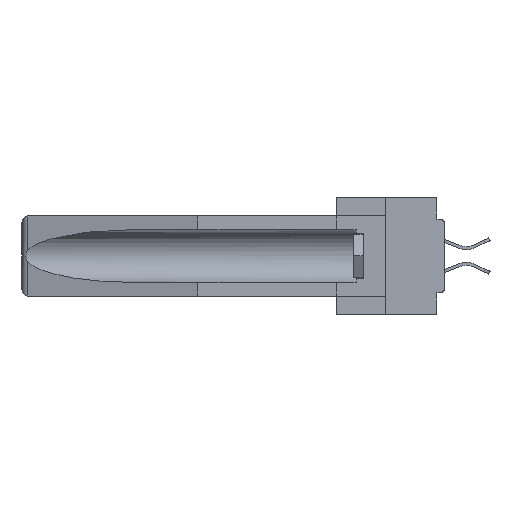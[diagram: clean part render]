
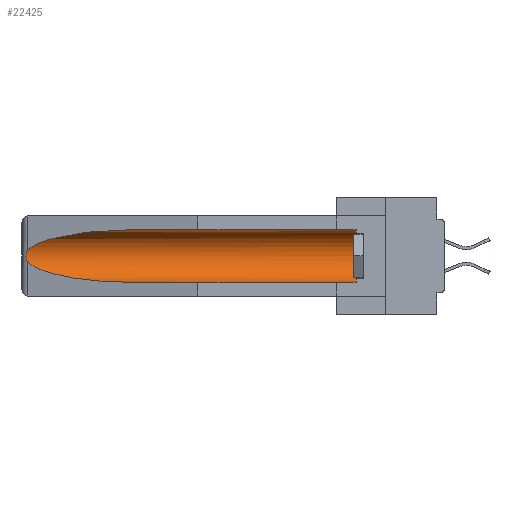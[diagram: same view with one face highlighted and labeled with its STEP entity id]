
A CAD part, left-side view. The second image highlights one B-rep face of the part: STEP entity #22425.
In plain terms, the highlighted cylindrical face has radius 2.857 mm (diameter 5.715 mm), a partial arc.
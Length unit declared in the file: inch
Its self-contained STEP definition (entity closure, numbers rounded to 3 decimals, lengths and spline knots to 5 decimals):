
#254 = CARTESIAN_POINT ( 'NONE',  ( 0.21114, 1.30732, -0.059 ) ) ;
#322 = EDGE_CURVE ( 'NONE', #24030, #15354, #25024, .T. ) ;
#728 = CARTESIAN_POINT ( 'NONE',  ( 0.2675, 1.53308, -0.16763 ) ) ;
#823 =( BOUNDED_CURVE ( )  B_SPLINE_CURVE ( 3, ( #20902, #254, #3367, #24155 ),
 .UNSPECIFIED., .F., .F. ) 
 B_SPLINE_CURVE_WITH_KNOTS ( ( 4, 4 ),
 ( 4.71239, 6.08839 ),
 .UNSPECIFIED. ) 
 CURVE ( )  GEOMETRIC_REPRESENTATION_ITEM ( )  RATIONAL_B_SPLINE_CURVE ( ( 1., 0.848, 0.848, 1. ) ) 
 REPRESENTATION_ITEM ( '' )  );
#825 = CYLINDRICAL_SURFACE ( 'NONE', #8034, 0.1125 ) ;
#1523 = B_SPLINE_CURVE_WITH_KNOTS ( 'NONE', 3,
 ( #2944, #11769, #5911, #36228, #728, #15561, #9840, #12424, #6300, #6419 ),
 .UNSPECIFIED., .F., .F.,
 ( 4, 2, 2, 2, 4 ),
 ( 0., 0.00029, 0.00058, 0.00087, 0.00117 ),
 .UNSPECIFIED. ) ;
#1564 = CARTESIAN_POINT ( 'NONE',  ( 0.155, -0.30754, -0.284 ) ) ;
#1683 = DIRECTION ( 'NONE',  ( 0., 1., 0. ) ) ;
#2037 = CARTESIAN_POINT ( 'NONE',  ( 0.155, 0.126, -0.1715 ) ) ;
#2944 = CARTESIAN_POINT ( 'NONE',  ( 0.26537, 1.52718, -0.14972 ) ) ;
#3367 = CARTESIAN_POINT ( 'NONE',  ( 0.25451, 1.48313, -0.09465 ) ) ;
#3453 = ORIENTED_EDGE ( 'NONE', *, *, #322, .T. ) ;
#4276 = VERTEX_POINT ( 'NONE', #21068 ) ;
#4538 = EDGE_LOOP ( 'NONE', ( #18793, #7656, #26432, #9390, #35405, #3453 ) ) ;
#5125 = CARTESIAN_POINT ( 'NONE',  ( 0.155, 1.07973, -0.284 ) ) ;
#5133 = DIRECTION ( 'NONE',  ( 0., 0., 1. ) ) ;
#5911 = CARTESIAN_POINT ( 'NONE',  ( 0.26654, 1.53092, -0.15636 ) ) ;
#6300 = CARTESIAN_POINT ( 'NONE',  ( 0.26597, 1.5296, -0.19026 ) ) ;
#6419 = CARTESIAN_POINT ( 'NONE',  ( 0.26537, 1.52718, -0.19328 ) ) ;
#6551 = DIRECTION ( 'NONE',  ( 0., 0., 1. ) ) ;
#6718 = CARTESIAN_POINT ( 'NONE',  ( 0.155, 1.07973, -0.059 ) ) ;
#7656 = ORIENTED_EDGE ( 'NONE', *, *, #36090, .T. ) ;
#8034 = AXIS2_PLACEMENT_3D ( 'NONE', #21124, #33382, #6551 ) ;
#9376 = CIRCLE ( 'NONE', #15101, 0.1125 ) ;
#9390 = ORIENTED_EDGE ( 'NONE', *, *, #18769, .F. ) ;
#9840 = CARTESIAN_POINT ( 'NONE',  ( 0.2673, 1.53269, -0.17917 ) ) ;
#11769 = CARTESIAN_POINT ( 'NONE',  ( 0.26597, 1.52961, -0.15275 ) ) ;
#12424 = CARTESIAN_POINT ( 'NONE',  ( 0.26655, 1.53094, -0.18657 ) ) ;
#12952 = CARTESIAN_POINT ( 'NONE',  ( 0.25451, 1.48313, -0.24835 ) ) ;
#13087 = CARTESIAN_POINT ( 'NONE',  ( 0.21114, 1.30732, -0.284 ) ) ;
#14111 = DIRECTION ( 'NONE',  ( 0., -1., 0. ) ) ;
#15101 = AXIS2_PLACEMENT_3D ( 'NONE', #2037, #14111, #5133 ) ;
#15354 = VERTEX_POINT ( 'NONE', #6718 ) ;
#15512 = CARTESIAN_POINT ( 'NONE',  ( 0.155, 0.126, -0.059 ) ) ;
#15561 = CARTESIAN_POINT ( 'NONE',  ( 0.2675, 1.53308, -0.17534 ) ) ;
#17628 = VECTOR ( 'NONE', #1683, 39.37008 ) ;
#18769 = EDGE_CURVE ( 'NONE', #21579, #19086, #25560, .T. ) ;
#18793 = ORIENTED_EDGE ( 'NONE', *, *, #18933, .T. ) ;
#18933 = EDGE_CURVE ( 'NONE', #15354, #36794, #823, .T. ) ;
#19086 = VERTEX_POINT ( 'NONE', #5125 ) ;
#20902 = CARTESIAN_POINT ( 'NONE',  ( 0.155, 1.07973, -0.059 ) ) ;
#21068 = CARTESIAN_POINT ( 'NONE',  ( 0.26537, 1.52718, -0.19328 ) ) ;
#21124 = CARTESIAN_POINT ( 'NONE',  ( 0.155, -0.30754, -0.1715 ) ) ;
#21579 = VERTEX_POINT ( 'NONE', #31750 ) ;
#21800 = CARTESIAN_POINT ( 'NONE',  ( 0.26537, 1.52718, -0.19328 ) ) ;
#22425 = ADVANCED_FACE ( 'NONE', ( #36643 ), #825, .F. ) ;
#23085 = VECTOR ( 'NONE', #34253, 39.37008 ) ;
#24030 = VERTEX_POINT ( 'NONE', #15512 ) ;
#24155 = CARTESIAN_POINT ( 'NONE',  ( 0.26537, 1.52718, -0.14972 ) ) ;
#25024 = LINE ( 'NONE', #33743, #23085 ) ;
#25560 = LINE ( 'NONE', #1564, #17628 ) ;
#25986 = EDGE_CURVE ( 'NONE', #4276, #19086, #29712, .T. ) ;
#26432 = ORIENTED_EDGE ( 'NONE', *, *, #25986, .T. ) ;
#29712 =( BOUNDED_CURVE ( )  B_SPLINE_CURVE ( 3, ( #21800, #12952, #13087, #36904 ),
 .UNSPECIFIED., .F., .F. ) 
 B_SPLINE_CURVE_WITH_KNOTS ( ( 4, 4 ),
 ( 0.1948, 1.5708 ),
 .UNSPECIFIED. ) 
 CURVE ( )  GEOMETRIC_REPRESENTATION_ITEM ( )  RATIONAL_B_SPLINE_CURVE ( ( 1., 0.848, 0.848, 1. ) ) 
 REPRESENTATION_ITEM ( '' )  );
#31750 = CARTESIAN_POINT ( 'NONE',  ( 0.155, 0.126, -0.284 ) ) ;
#33382 = DIRECTION ( 'NONE',  ( 0., 1., 0. ) ) ;
#33743 = CARTESIAN_POINT ( 'NONE',  ( 0.155, -0.30754, -0.059 ) ) ;
#34253 = DIRECTION ( 'NONE',  ( 0., 1., 0. ) ) ;
#35405 = ORIENTED_EDGE ( 'NONE', *, *, #35875, .T. ) ;
#35875 = EDGE_CURVE ( 'NONE', #21579, #24030, #9376, .T. ) ;
#36090 = EDGE_CURVE ( 'NONE', #36794, #4276, #1523, .T. ) ;
#36228 = CARTESIAN_POINT ( 'NONE',  ( 0.2673, 1.5327, -0.16383 ) ) ;
#36643 = FACE_OUTER_BOUND ( 'NONE', #4538, .T. ) ;
#36794 = VERTEX_POINT ( 'NONE', #37976 ) ;
#36904 = CARTESIAN_POINT ( 'NONE',  ( 0.155, 1.07973, -0.284 ) ) ;
#37976 = CARTESIAN_POINT ( 'NONE',  ( 0.26537, 1.52718, -0.14972 ) ) ;
